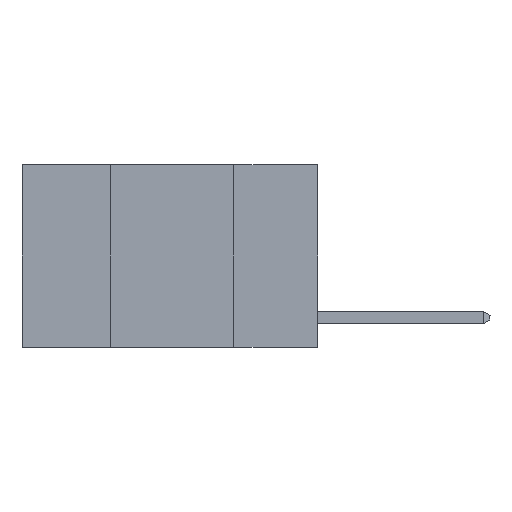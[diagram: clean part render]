
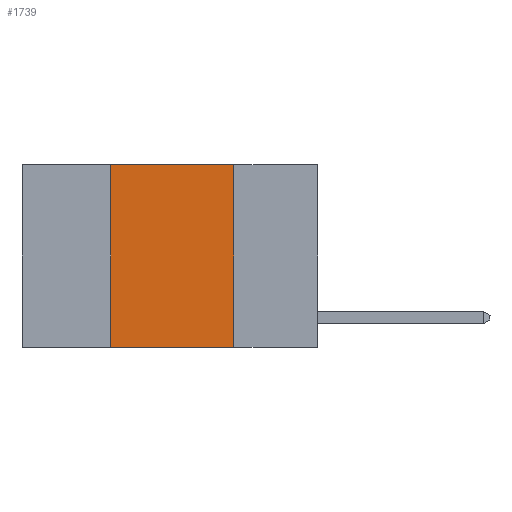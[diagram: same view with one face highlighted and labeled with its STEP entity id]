
A CAD part, left-side view. The second image highlights one B-rep face of the part: STEP entity #1739.
In plain terms, the highlighted planar face has unit normal (-1, 0, 0).
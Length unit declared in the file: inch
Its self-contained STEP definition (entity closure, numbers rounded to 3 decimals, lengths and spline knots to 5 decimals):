
#417 = VERTEX_POINT ( 'NONE', #6915 ) ;
#953 = PLANE ( 'NONE',  #10752 ) ;
#964 = VERTEX_POINT ( 'NONE', #9300 ) ;
#1506 = CARTESIAN_POINT ( 'NONE',  ( 0., 0.42, -0.37 ) ) ;
#1739 = ADVANCED_FACE ( 'NONE', ( #8230 ), #953, .F. ) ;
#1909 = LINE ( 'NONE', #4205, #4106 ) ;
#2221 = EDGE_CURVE ( 'NONE', #417, #11142, #1909, .T. ) ;
#2392 = CARTESIAN_POINT ( 'NONE',  ( 0., 0.6, -0.37 ) ) ;
#2850 = ORIENTED_EDGE ( 'NONE', *, *, #4516, .F. ) ;
#3365 = DIRECTION ( 'NONE',  ( 0., -1., 0. ) ) ;
#3609 = VECTOR ( 'NONE', #9457, 39.37008 ) ;
#3788 = VERTEX_POINT ( 'NONE', #1506 ) ;
#3883 = ORIENTED_EDGE ( 'NONE', *, *, #9091, .T. ) ;
#4106 = VECTOR ( 'NONE', #10357, 39.37008 ) ;
#4205 = CARTESIAN_POINT ( 'NONE',  ( 0., 0.6, 0. ) ) ;
#4516 = EDGE_CURVE ( 'NONE', #11142, #964, #10090, .T. ) ;
#4562 = LINE ( 'NONE', #10188, #3609 ) ;
#4767 = ORIENTED_EDGE ( 'NONE', *, *, #2221, .F. ) ;
#5454 = DIRECTION ( 'NONE',  ( 0., 0., -1. ) ) ;
#6004 = CARTESIAN_POINT ( 'NONE',  ( 0., 0.17, 0. ) ) ;
#6182 = VECTOR ( 'NONE', #3365, 39.37008 ) ;
#6236 = EDGE_CURVE ( 'NONE', #3788, #417, #4562, .T. ) ;
#6915 = CARTESIAN_POINT ( 'NONE',  ( 0., 0.42, 0. ) ) ;
#7338 = CARTESIAN_POINT ( 'NONE',  ( 0., 0.17, 0. ) ) ;
#8230 = FACE_OUTER_BOUND ( 'NONE', #11057, .T. ) ;
#8468 = DIRECTION ( 'NONE',  ( 0., 0., -1. ) ) ;
#8643 = ORIENTED_EDGE ( 'NONE', *, *, #6236, .F. ) ;
#8944 = CARTESIAN_POINT ( 'NONE',  ( 0., 0.6, 0. ) ) ;
#9091 = EDGE_CURVE ( 'NONE', #3788, #964, #10002, .T. ) ;
#9300 = CARTESIAN_POINT ( 'NONE',  ( 0., 0.17, -0.37 ) ) ;
#9457 = DIRECTION ( 'NONE',  ( 0., 0., 1. ) ) ;
#9548 = VECTOR ( 'NONE', #8468, 39.37008 ) ;
#10002 = LINE ( 'NONE', #2392, #6182 ) ;
#10090 = LINE ( 'NONE', #6004, #9548 ) ;
#10188 = CARTESIAN_POINT ( 'NONE',  ( 0., 0.42, 0. ) ) ;
#10357 = DIRECTION ( 'NONE',  ( 0., -1., 0. ) ) ;
#10700 = DIRECTION ( 'NONE',  ( 1., 0., 0. ) ) ;
#10752 = AXIS2_PLACEMENT_3D ( 'NONE', #8944, #10700, #5454 ) ;
#11057 = EDGE_LOOP ( 'NONE', ( #2850, #4767, #8643, #3883 ) ) ;
#11142 = VERTEX_POINT ( 'NONE', #7338 ) ;
